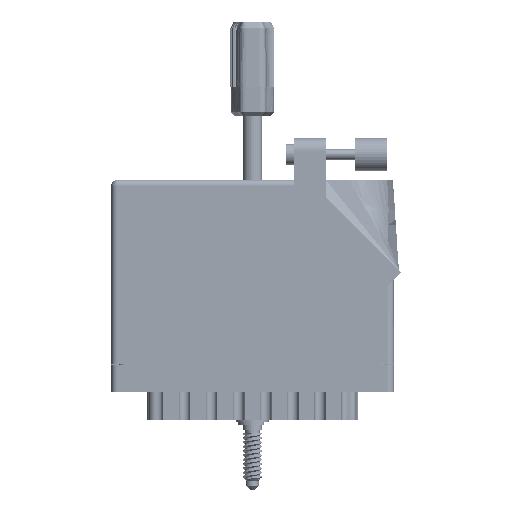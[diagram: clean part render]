
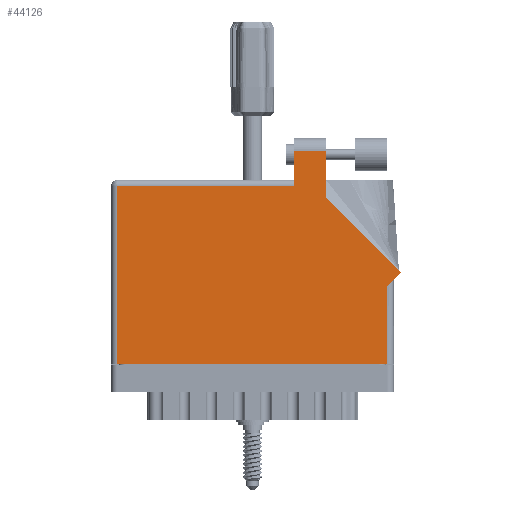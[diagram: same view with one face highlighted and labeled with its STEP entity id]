
A CAD part, front view. The second image highlights one B-rep face of the part: STEP entity #44126.
In plain terms, the highlighted face is planar.
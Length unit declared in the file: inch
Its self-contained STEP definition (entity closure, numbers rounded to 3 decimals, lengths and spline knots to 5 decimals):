
#1657 = ORIENTED_EDGE ( 'NONE', *, *, #80984, .T. ) ;
#2702 = CARTESIAN_POINT ( 'NONE',  ( 0., 1.775, 0. ) ) ;
#2942 = VECTOR ( 'NONE', #86790, 39.37008 ) ;
#3111 = ORIENTED_EDGE ( 'NONE', *, *, #10686, .T. ) ;
#3230 = CARTESIAN_POINT ( 'NONE',  ( 2.656, 0.753, 0. ) ) ;
#7859 = CARTESIAN_POINT ( 'NONE',  ( 2.656, 0.815, 0. ) ) ;
#10189 = VERTEX_POINT ( 'NONE', #13494 ) ;
#10686 = EDGE_CURVE ( 'NONE', #10189, #78951, #21290, .T. ) ;
#10761 = CARTESIAN_POINT ( 'NONE',  ( 0.062, 1.713, 0. ) ) ;
#11232 = EDGE_CURVE ( 'NONE', #76277, #71943, #70956, .T. ) ;
#11537 = CARTESIAN_POINT ( 'NONE',  ( 2.065, 1.60942, 0. ) ) ;
#13207 = EDGE_CURVE ( 'NONE', #71943, #52156, #48100, .T. ) ;
#13494 = CARTESIAN_POINT ( 'NONE',  ( 2.78871, 0.88571, 0. ) ) ;
#14468 = LINE ( 'NONE', #7859, #74968 ) ;
#15096 = VECTOR ( 'NONE', #18681, 39.37008 ) ;
#15575 = VECTOR ( 'NONE', #65106, 39.37008 ) ;
#18170 = LINE ( 'NONE', #11537, #75501 ) ;
#18681 = DIRECTION ( 'NONE',  ( 0., -1., 0. ) ) ;
#19156 = EDGE_CURVE ( 'NONE', #52156, #80262, #46023, .T. ) ;
#19568 = CARTESIAN_POINT ( 'NONE',  ( 0.062, 0., 0. ) ) ;
#20974 = LINE ( 'NONE', #58225, #45839 ) ;
#21290 = LINE ( 'NONE', #73815, #2942 ) ;
#22034 = ORIENTED_EDGE ( 'NONE', *, *, #29924, .T. ) ;
#22792 = EDGE_LOOP ( 'NONE', ( #1657, #27233, #26547, #31726, #80530, #71537, #32032, #22034, #3111 ) ) ;
#23511 = DIRECTION ( 'NONE',  ( 0., 0., -1. ) ) ;
#26547 = ORIENTED_EDGE ( 'NONE', *, *, #13207, .T. ) ;
#27233 = ORIENTED_EDGE ( 'NONE', *, *, #11232, .T. ) ;
#28328 = FACE_OUTER_BOUND ( 'NONE', #22792, .T. ) ;
#29487 = CARTESIAN_POINT ( 'NONE',  ( 2.718, 0.815, 0. ) ) ;
#29924 = EDGE_CURVE ( 'NONE', #49814, #10189, #38470, .T. ) ;
#30125 = DIRECTION ( 'NONE',  ( 1., 0., 0. ) ) ;
#31726 = ORIENTED_EDGE ( 'NONE', *, *, #19156, .T. ) ;
#32032 = ORIENTED_EDGE ( 'NONE', *, *, #59916, .T. ) ;
#32322 = CARTESIAN_POINT ( 'NONE',  ( 2.065, 2.05, 0. ) ) ;
#36156 = DIRECTION ( 'NONE',  ( 0.707, 0.707, 0. ) ) ;
#38470 = LINE ( 'NONE', #29487, #67509 ) ;
#38949 = DIRECTION ( 'NONE',  ( -1., 0., 0. ) ) ;
#44073 = PLANE ( 'NONE',  #56161 ) ;
#44126 = ADVANCED_FACE ( 'NONE', ( #28328 ), #44073, .F. ) ;
#45646 = CARTESIAN_POINT ( 'NONE',  ( 1.758, 2.05, 0. ) ) ;
#45687 = VERTEX_POINT ( 'NONE', #56056 ) ;
#45839 = VECTOR ( 'NONE', #30125, 39.37008 ) ;
#46023 = LINE ( 'NONE', #87479, #87070 ) ;
#46241 = VERTEX_POINT ( 'NONE', #62283 ) ;
#48100 = LINE ( 'NONE', #85935, #15575 ) ;
#49814 = VERTEX_POINT ( 'NONE', #3230 ) ;
#50098 = DIRECTION ( 'NONE',  ( 0., 1., 0. ) ) ;
#52156 = VERTEX_POINT ( 'NONE', #58656 ) ;
#52294 = DIRECTION ( 'NONE',  ( -1., 0., 0. ) ) ;
#52575 = VECTOR ( 'NONE', #52294, 39.37008 ) ;
#56056 = CARTESIAN_POINT ( 'NONE',  ( 0.062, 0., 0. ) ) ;
#56106 = LINE ( 'NONE', #19568, #15096 ) ;
#56161 = AXIS2_PLACEMENT_3D ( 'NONE', #2702, #23511, #65475 ) ;
#58225 = CARTESIAN_POINT ( 'NONE',  ( 0., 0., 0. ) ) ;
#58656 = CARTESIAN_POINT ( 'NONE',  ( 1.758, 1.713, 0. ) ) ;
#59916 = EDGE_CURVE ( 'NONE', #46241, #49814, #14468, .T. ) ;
#62283 = CARTESIAN_POINT ( 'NONE',  ( 2.656, 0., 0. ) ) ;
#65106 = DIRECTION ( 'NONE',  ( 0., -1., 0. ) ) ;
#65475 = DIRECTION ( 'NONE',  ( -1., 0., 0. ) ) ;
#67085 = DIRECTION ( 'NONE',  ( 0., 1., 0. ) ) ;
#67509 = VECTOR ( 'NONE', #36156, 39.37008 ) ;
#70956 = LINE ( 'NONE', #45646, #52575 ) ;
#71537 = ORIENTED_EDGE ( 'NONE', *, *, #77784, .T. ) ;
#71943 = VERTEX_POINT ( 'NONE', #87434 ) ;
#73177 = EDGE_CURVE ( 'NONE', #80262, #45687, #56106, .T. ) ;
#73815 = CARTESIAN_POINT ( 'NONE',  ( 2.78871, 0.88571, 0. ) ) ;
#74968 = VECTOR ( 'NONE', #50098, 39.37008 ) ;
#75501 = VECTOR ( 'NONE', #67085, 39.37008 ) ;
#76277 = VERTEX_POINT ( 'NONE', #32322 ) ;
#77068 = CARTESIAN_POINT ( 'NONE',  ( 2.065, 1.60942, 0. ) ) ;
#77784 = EDGE_CURVE ( 'NONE', #45687, #46241, #20974, .T. ) ;
#78951 = VERTEX_POINT ( 'NONE', #77068 ) ;
#80262 = VERTEX_POINT ( 'NONE', #10761 ) ;
#80530 = ORIENTED_EDGE ( 'NONE', *, *, #73177, .T. ) ;
#80984 = EDGE_CURVE ( 'NONE', #78951, #76277, #18170, .T. ) ;
#85935 = CARTESIAN_POINT ( 'NONE',  ( 1.758, 1.775, 0. ) ) ;
#86790 = DIRECTION ( 'NONE',  ( -0.707, 0.707, 0. ) ) ;
#87070 = VECTOR ( 'NONE', #38949, 39.37008 ) ;
#87434 = CARTESIAN_POINT ( 'NONE',  ( 1.758, 2.05, 0. ) ) ;
#87479 = CARTESIAN_POINT ( 'NONE',  ( 0., 1.713, 0. ) ) ;
